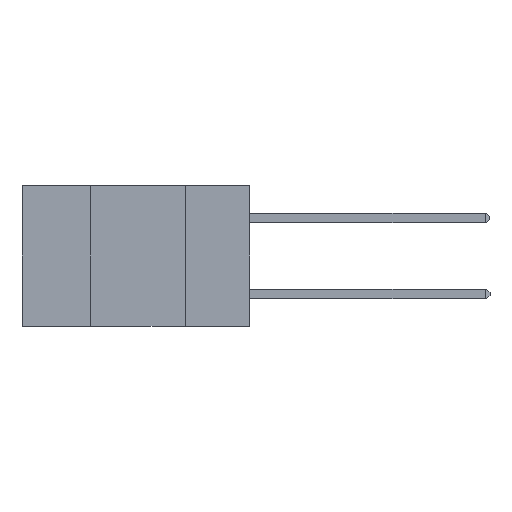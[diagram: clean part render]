
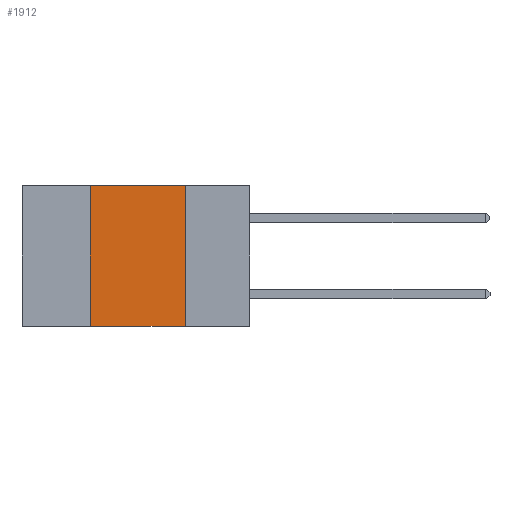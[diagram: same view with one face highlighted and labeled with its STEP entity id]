
A CAD part, left-side view. The second image highlights one B-rep face of the part: STEP entity #1912.
In plain terms, the highlighted planar face has unit normal (-1, 0, 0).
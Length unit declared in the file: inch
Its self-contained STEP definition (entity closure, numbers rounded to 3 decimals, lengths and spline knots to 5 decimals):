
#164 = DIRECTION ( 'NONE',  ( 0., -1., 0. ) ) ;
#951 = VECTOR ( 'NONE', #6441, 39.37008 ) ;
#992 = CARTESIAN_POINT ( 'NONE',  ( 0., 0.17, -0.37 ) ) ;
#1459 = CARTESIAN_POINT ( 'NONE',  ( 0., 0.6, -0.37 ) ) ;
#1473 = LINE ( 'NONE', #6273, #8695 ) ;
#1912 = ADVANCED_FACE ( 'NONE', ( #11620 ), #11093, .F. ) ;
#2583 = DIRECTION ( 'NONE',  ( 0., 0., -1. ) ) ;
#2629 = VECTOR ( 'NONE', #4013, 39.37008 ) ;
#2803 = CARTESIAN_POINT ( 'NONE',  ( 0., 0.42, 0. ) ) ;
#3155 = VERTEX_POINT ( 'NONE', #992 ) ;
#3203 = ORIENTED_EDGE ( 'NONE', *, *, #3979, .T. ) ;
#3506 = EDGE_LOOP ( 'NONE', ( #11341, #7190, #7774, #3203 ) ) ;
#3839 = VECTOR ( 'NONE', #164, 39.37008 ) ;
#3979 = EDGE_CURVE ( 'NONE', #7856, #3155, #5056, .T. ) ;
#4013 = DIRECTION ( 'NONE',  ( 0., -1., 0. ) ) ;
#4217 = DIRECTION ( 'NONE',  ( 0., 0., -1. ) ) ;
#4901 = CARTESIAN_POINT ( 'NONE',  ( 0., 0.6, 0. ) ) ;
#5056 = LINE ( 'NONE', #1459, #2629 ) ;
#5824 = VERTEX_POINT ( 'NONE', #10084 ) ;
#6250 = LINE ( 'NONE', #8314, #3839 ) ;
#6270 = VERTEX_POINT ( 'NONE', #10667 ) ;
#6273 = CARTESIAN_POINT ( 'NONE',  ( 0., 0.17, 0. ) ) ;
#6441 = DIRECTION ( 'NONE',  ( 0., 0., 1. ) ) ;
#7190 = ORIENTED_EDGE ( 'NONE', *, *, #8950, .F. ) ;
#7651 = EDGE_CURVE ( 'NONE', #5824, #3155, #1473, .T. ) ;
#7774 = ORIENTED_EDGE ( 'NONE', *, *, #11400, .F. ) ;
#7856 = VERTEX_POINT ( 'NONE', #8375 ) ;
#8314 = CARTESIAN_POINT ( 'NONE',  ( 0., 0.6, 0. ) ) ;
#8375 = CARTESIAN_POINT ( 'NONE',  ( 0., 0.42, -0.37 ) ) ;
#8459 = LINE ( 'NONE', #2803, #951 ) ;
#8695 = VECTOR ( 'NONE', #2583, 39.37008 ) ;
#8901 = AXIS2_PLACEMENT_3D ( 'NONE', #4901, #10279, #4217 ) ;
#8950 = EDGE_CURVE ( 'NONE', #6270, #5824, #6250, .T. ) ;
#10084 = CARTESIAN_POINT ( 'NONE',  ( 0., 0.17, 0. ) ) ;
#10279 = DIRECTION ( 'NONE',  ( 1., 0., 0. ) ) ;
#10667 = CARTESIAN_POINT ( 'NONE',  ( 0., 0.42, 0. ) ) ;
#11093 = PLANE ( 'NONE',  #8901 ) ;
#11341 = ORIENTED_EDGE ( 'NONE', *, *, #7651, .F. ) ;
#11400 = EDGE_CURVE ( 'NONE', #7856, #6270, #8459, .T. ) ;
#11620 = FACE_OUTER_BOUND ( 'NONE', #3506, .T. ) ;
